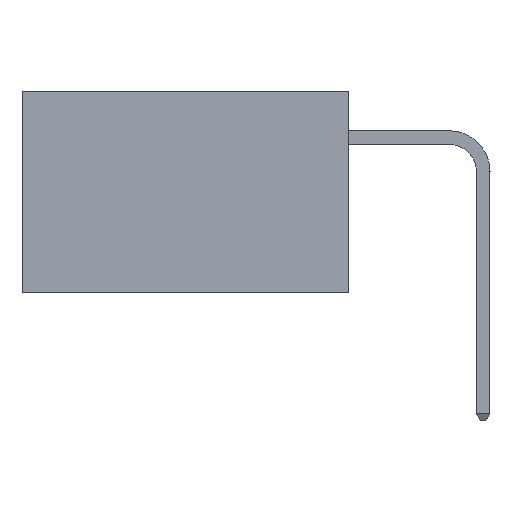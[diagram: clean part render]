
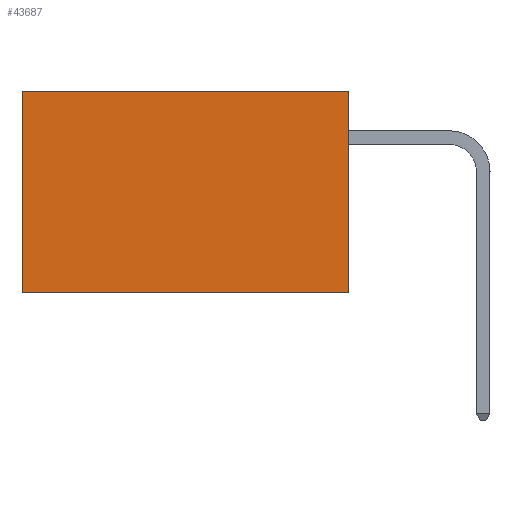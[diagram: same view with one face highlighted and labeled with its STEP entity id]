
A CAD part, left-side view. The second image highlights one B-rep face of the part: STEP entity #43687.
In plain terms, the highlighted planar face has unit normal (-1, 0, 0).
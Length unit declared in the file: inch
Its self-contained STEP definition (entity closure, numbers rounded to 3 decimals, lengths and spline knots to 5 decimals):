
#1245 = DIRECTION ( 'NONE',  ( 1., 0., 0. ) ) ;
#4261 = AXIS2_PLACEMENT_3D ( 'NONE', #23519, #1245, #27234 ) ;
#4939 = VECTOR ( 'NONE', #45713, 39.37008 ) ;
#9707 = DIRECTION ( 'NONE',  ( 0., 0., -1. ) ) ;
#10655 = LINE ( 'NONE', #31878, #29164 ) ;
#13551 = DIRECTION ( 'NONE',  ( 0., 1., 0. ) ) ;
#15865 = CARTESIAN_POINT ( 'NONE',  ( 0.2875, 0.6, -0.37 ) ) ;
#15980 = EDGE_CURVE ( 'NONE', #38632, #31476, #20593, .T. ) ;
#17704 = EDGE_CURVE ( 'NONE', #31476, #39897, #37751, .T. ) ;
#17944 = DIRECTION ( 'NONE',  ( 0., 0., -1. ) ) ;
#18688 = CARTESIAN_POINT ( 'NONE',  ( 0.2875, 0.6, 0. ) ) ;
#18781 = CARTESIAN_POINT ( 'NONE',  ( 0.2875, 0., -0.37 ) ) ;
#19352 = VERTEX_POINT ( 'NONE', #18688 ) ;
#19422 = VECTOR ( 'NONE', #17944, 39.37008 ) ;
#19792 = CARTESIAN_POINT ( 'NONE',  ( 0.2875, 0., 0. ) ) ;
#20593 = LINE ( 'NONE', #36526, #19422 ) ;
#21144 = EDGE_LOOP ( 'NONE', ( #36698, #45712, #29922, #31061 ) ) ;
#21235 = LINE ( 'NONE', #19792, #4939 ) ;
#23519 = CARTESIAN_POINT ( 'NONE',  ( 0.2875, 0., 0. ) ) ;
#26836 = CARTESIAN_POINT ( 'NONE',  ( 0.2875, 0., 0. ) ) ;
#27234 = DIRECTION ( 'NONE',  ( 0., 0., -1. ) ) ;
#28570 = EDGE_CURVE ( 'NONE', #19352, #39897, #10655, .T. ) ;
#29164 = VECTOR ( 'NONE', #9707, 39.37008 ) ;
#29922 = ORIENTED_EDGE ( 'NONE', *, *, #15980, .F. ) ;
#30228 = VECTOR ( 'NONE', #13551, 39.37008 ) ;
#31061 = ORIENTED_EDGE ( 'NONE', *, *, #47175, .T. ) ;
#31476 = VERTEX_POINT ( 'NONE', #18781 ) ;
#31878 = CARTESIAN_POINT ( 'NONE',  ( 0.2875, 0.6, 0. ) ) ;
#35729 = CARTESIAN_POINT ( 'NONE',  ( 0.2875, 0., -0.37 ) ) ;
#36526 = CARTESIAN_POINT ( 'NONE',  ( 0.2875, 0., 0. ) ) ;
#36698 = ORIENTED_EDGE ( 'NONE', *, *, #28570, .T. ) ;
#37751 = LINE ( 'NONE', #35729, #30228 ) ;
#38632 = VERTEX_POINT ( 'NONE', #26836 ) ;
#39897 = VERTEX_POINT ( 'NONE', #15865 ) ;
#40108 = FACE_OUTER_BOUND ( 'NONE', #21144, .T. ) ;
#43687 = ADVANCED_FACE ( 'NONE', ( #40108 ), #45592, .F. ) ;
#45592 = PLANE ( 'NONE',  #4261 ) ;
#45712 = ORIENTED_EDGE ( 'NONE', *, *, #17704, .F. ) ;
#45713 = DIRECTION ( 'NONE',  ( 0., 1., 0. ) ) ;
#47175 = EDGE_CURVE ( 'NONE', #38632, #19352, #21235, .T. ) ;
